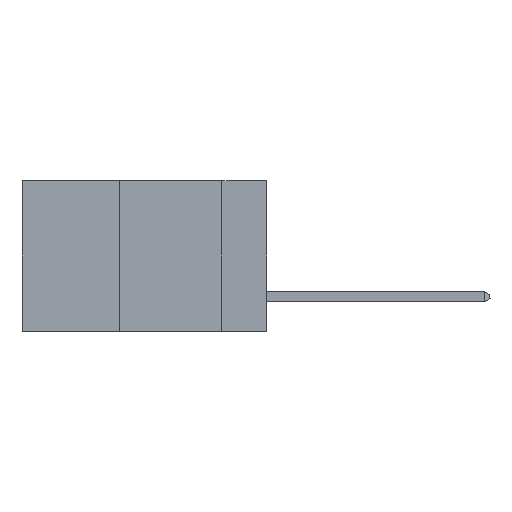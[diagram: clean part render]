
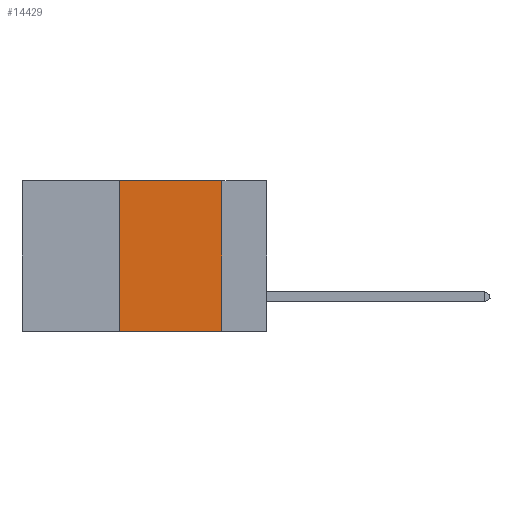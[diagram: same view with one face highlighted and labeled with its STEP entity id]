
A CAD part, left-side view. The second image highlights one B-rep face of the part: STEP entity #14429.
In plain terms, the highlighted planar face has unit normal (-1, 0, 0).
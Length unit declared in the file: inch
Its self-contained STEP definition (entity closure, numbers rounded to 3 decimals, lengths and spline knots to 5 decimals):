
#230 = VERTEX_POINT ( 'NONE', #34246 ) ;
#632 = LINE ( 'NONE', #19990, #37404 ) ;
#1554 = FACE_OUTER_BOUND ( 'NONE', #10522, .T. ) ;
#3202 = VERTEX_POINT ( 'NONE', #3288 ) ;
#3288 = CARTESIAN_POINT ( 'NONE',  ( 0., 0.11, 0. ) ) ;
#4939 = CARTESIAN_POINT ( 'NONE',  ( 0., 0.11, -0.37 ) ) ;
#8399 = AXIS2_PLACEMENT_3D ( 'NONE', #12550, #23980, #37434 ) ;
#8879 = LINE ( 'NONE', #45490, #34519 ) ;
#9662 = DIRECTION ( 'NONE',  ( 0., 0., 1. ) ) ;
#9863 = VECTOR ( 'NONE', #44136, 39.37008 ) ;
#10522 = EDGE_LOOP ( 'NONE', ( #23514, #27836, #31791, #17793 ) ) ;
#12550 = CARTESIAN_POINT ( 'NONE',  ( 0., 0.6, 0. ) ) ;
#13193 = PLANE ( 'NONE',  #8399 ) ;
#14429 = ADVANCED_FACE ( 'NONE', ( #1554 ), #13193, .F. ) ;
#14579 = EDGE_CURVE ( 'NONE', #3202, #21323, #19330, .T. ) ;
#16700 = VECTOR ( 'NONE', #31503, 39.37008 ) ;
#17793 = ORIENTED_EDGE ( 'NONE', *, *, #39383, .T. ) ;
#19330 = LINE ( 'NONE', #36720, #9863 ) ;
#19990 = CARTESIAN_POINT ( 'NONE',  ( 0., 0.6, 0. ) ) ;
#21323 = VERTEX_POINT ( 'NONE', #4939 ) ;
#22741 = DIRECTION ( 'NONE',  ( 0., -1., 0. ) ) ;
#23514 = ORIENTED_EDGE ( 'NONE', *, *, #14579, .F. ) ;
#23980 = DIRECTION ( 'NONE',  ( 1., 0., 0. ) ) ;
#24543 = EDGE_CURVE ( 'NONE', #38609, #230, #8879, .T. ) ;
#27836 = ORIENTED_EDGE ( 'NONE', *, *, #34028, .F. ) ;
#31199 = CARTESIAN_POINT ( 'NONE',  ( 0., 0.6, -0.37 ) ) ;
#31503 = DIRECTION ( 'NONE',  ( 0., -1., 0. ) ) ;
#31791 = ORIENTED_EDGE ( 'NONE', *, *, #24543, .F. ) ;
#34028 = EDGE_CURVE ( 'NONE', #230, #3202, #632, .T. ) ;
#34246 = CARTESIAN_POINT ( 'NONE',  ( 0., 0.36, 0. ) ) ;
#34519 = VECTOR ( 'NONE', #9662, 39.37008 ) ;
#36720 = CARTESIAN_POINT ( 'NONE',  ( 0., 0.11, 0. ) ) ;
#37404 = VECTOR ( 'NONE', #22741, 39.37008 ) ;
#37434 = DIRECTION ( 'NONE',  ( 0., 0., -1. ) ) ;
#38392 = LINE ( 'NONE', #31199, #16700 ) ;
#38609 = VERTEX_POINT ( 'NONE', #41482 ) ;
#39383 = EDGE_CURVE ( 'NONE', #38609, #21323, #38392, .T. ) ;
#41482 = CARTESIAN_POINT ( 'NONE',  ( 0., 0.36, -0.37 ) ) ;
#44136 = DIRECTION ( 'NONE',  ( 0., 0., -1. ) ) ;
#45490 = CARTESIAN_POINT ( 'NONE',  ( 0., 0.36, 0. ) ) ;
